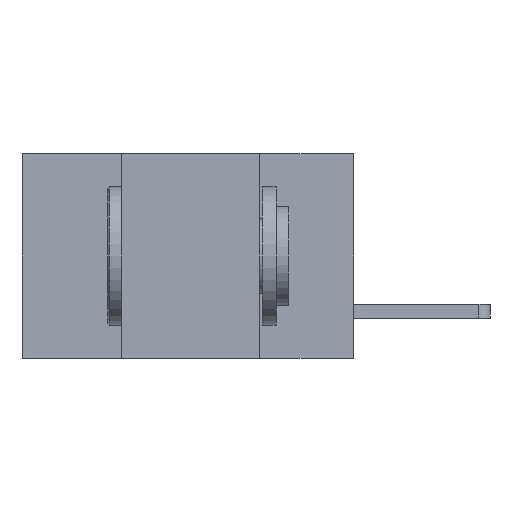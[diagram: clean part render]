
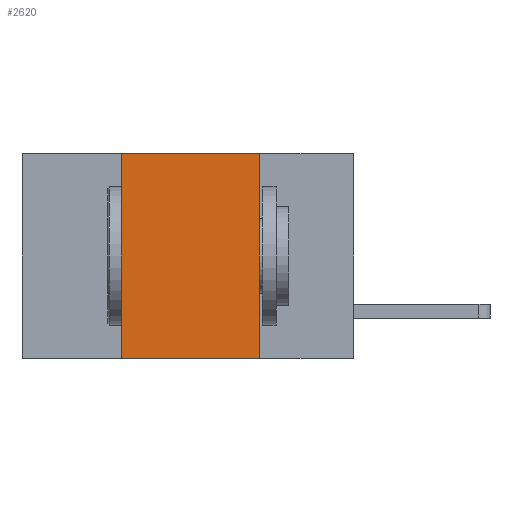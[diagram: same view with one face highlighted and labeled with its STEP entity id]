
A CAD part, left-side view. The second image highlights one B-rep face of the part: STEP entity #2620.
In plain terms, the highlighted planar face has unit normal (-1, 0, 0).
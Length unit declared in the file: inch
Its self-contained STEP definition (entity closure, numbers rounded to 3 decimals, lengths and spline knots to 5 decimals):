
#36 = EDGE_CURVE ( 'NONE', #3118, #615, #4309, .T. ) ;
#471 = DIRECTION ( 'NONE',  ( 1., 0., 0. ) ) ;
#615 = VERTEX_POINT ( 'NONE', #4001 ) ;
#1157 = CARTESIAN_POINT ( 'NONE',  ( 0., 0.42, 0. ) ) ;
#1187 = CARTESIAN_POINT ( 'NONE',  ( 0., 0.6, 0. ) ) ;
#1289 = AXIS2_PLACEMENT_3D ( 'NONE', #1187, #471, #9243 ) ;
#1612 = DIRECTION ( 'NONE',  ( 0., -1., 0. ) ) ;
#1982 = CARTESIAN_POINT ( 'NONE',  ( 0., 0.42, 0. ) ) ;
#2127 = VECTOR ( 'NONE', #3429, 39.37008 ) ;
#2281 = VERTEX_POINT ( 'NONE', #1157 ) ;
#2458 = VECTOR ( 'NONE', #2921, 39.37008 ) ;
#2482 = ORIENTED_EDGE ( 'NONE', *, *, #6168, .F. ) ;
#2553 = LINE ( 'NONE', #1982, #8670 ) ;
#2620 = ADVANCED_FACE ( 'NONE', ( #7077 ), #7753, .F. ) ;
#2921 = DIRECTION ( 'NONE',  ( 0., -1., 0. ) ) ;
#3118 = VERTEX_POINT ( 'NONE', #6573 ) ;
#3429 = DIRECTION ( 'NONE',  ( 0., 0., -1. ) ) ;
#4001 = CARTESIAN_POINT ( 'NONE',  ( 0., 0.17, -0.37 ) ) ;
#4309 = LINE ( 'NONE', #8059, #2458 ) ;
#4662 = VERTEX_POINT ( 'NONE', #7968 ) ;
#4903 = DIRECTION ( 'NONE',  ( 0., 0., 1. ) ) ;
#5256 = ORIENTED_EDGE ( 'NONE', *, *, #5653, .F. ) ;
#5530 = EDGE_LOOP ( 'NONE', ( #8374, #5256, #2482, #8187 ) ) ;
#5653 = EDGE_CURVE ( 'NONE', #2281, #4662, #7558, .T. ) ;
#5768 = VECTOR ( 'NONE', #1612, 39.37008 ) ;
#6168 = EDGE_CURVE ( 'NONE', #3118, #2281, #2553, .T. ) ;
#6395 = LINE ( 'NONE', #7166, #2127 ) ;
#6573 = CARTESIAN_POINT ( 'NONE',  ( 0., 0.42, -0.37 ) ) ;
#7077 = FACE_OUTER_BOUND ( 'NONE', #5530, .T. ) ;
#7166 = CARTESIAN_POINT ( 'NONE',  ( 0., 0.17, 0. ) ) ;
#7558 = LINE ( 'NONE', #8178, #5768 ) ;
#7753 = PLANE ( 'NONE',  #1289 ) ;
#7879 = EDGE_CURVE ( 'NONE', #4662, #615, #6395, .T. ) ;
#7968 = CARTESIAN_POINT ( 'NONE',  ( 0., 0.17, 0. ) ) ;
#8059 = CARTESIAN_POINT ( 'NONE',  ( 0., 0.6, -0.37 ) ) ;
#8178 = CARTESIAN_POINT ( 'NONE',  ( 0., 0.6, 0. ) ) ;
#8187 = ORIENTED_EDGE ( 'NONE', *, *, #36, .T. ) ;
#8374 = ORIENTED_EDGE ( 'NONE', *, *, #7879, .F. ) ;
#8670 = VECTOR ( 'NONE', #4903, 39.37008 ) ;
#9243 = DIRECTION ( 'NONE',  ( 0., 0., -1. ) ) ;
